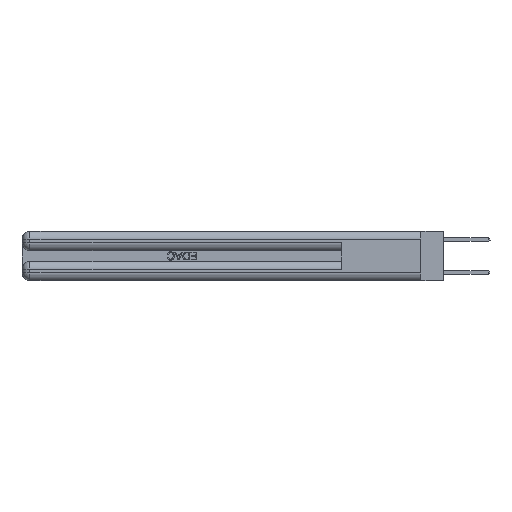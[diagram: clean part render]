
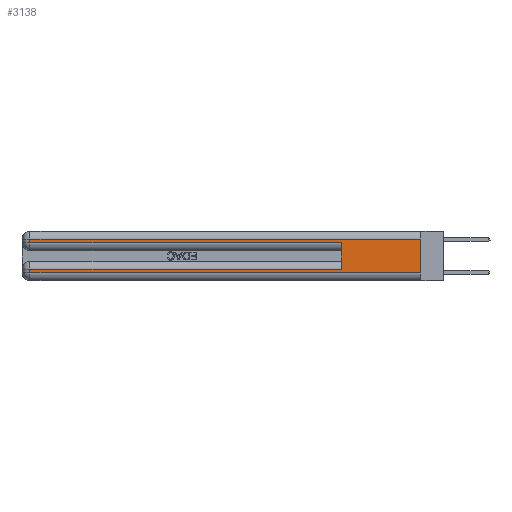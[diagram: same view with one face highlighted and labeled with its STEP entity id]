
A CAD part, left-side view. The second image highlights one B-rep face of the part: STEP entity #3138.
In plain terms, the highlighted planar face has unit normal (-1, 0, 0).
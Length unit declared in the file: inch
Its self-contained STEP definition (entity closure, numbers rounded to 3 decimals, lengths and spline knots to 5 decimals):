
#809 = VECTOR ( 'NONE', #23905, 39.37008 ) ;
#1511 = DIRECTION ( 'NONE',  ( 0., 1., 0. ) ) ;
#3138 = ADVANCED_FACE ( 'NONE', ( #25318 ), #23075, .F. ) ;
#3293 = LINE ( 'NONE', #7125, #24920 ) ;
#3451 = EDGE_CURVE ( 'NONE', #7905, #27086, #21387, .T. ) ;
#3602 = ORIENTED_EDGE ( 'NONE', *, *, #33795, .F. ) ;
#3707 = DIRECTION ( 'NONE',  ( 0., 0., -1. ) ) ;
#3880 = LINE ( 'NONE', #6873, #10560 ) ;
#3976 = CARTESIAN_POINT ( 'NONE',  ( 0., 2.94, 0.085 ) ) ;
#4169 = CARTESIAN_POINT ( 'NONE',  ( 0., 0., 0.285 ) ) ;
#4505 = VERTEX_POINT ( 'NONE', #17745 ) ;
#5614 = EDGE_CURVE ( 'NONE', #29169, #7905, #15104, .T. ) ;
#6213 = DIRECTION ( 'NONE',  ( 1., 0., 0. ) ) ;
#6358 = CARTESIAN_POINT ( 'NONE',  ( 0., 0., 0.06 ) ) ;
#6873 = CARTESIAN_POINT ( 'NONE',  ( 0., 2.94, 0.37 ) ) ;
#7125 = CARTESIAN_POINT ( 'NONE',  ( 0., 0., 0.31 ) ) ;
#7577 = VECTOR ( 'NONE', #28096, 39.37008 ) ;
#7658 = ORIENTED_EDGE ( 'NONE', *, *, #3451, .T. ) ;
#7905 = VERTEX_POINT ( 'NONE', #3976 ) ;
#7918 = EDGE_CURVE ( 'NONE', #4505, #29304, #3880, .T. ) ;
#8429 = ORIENTED_EDGE ( 'NONE', *, *, #30486, .T. ) ;
#9178 = DIRECTION ( 'NONE',  ( 0., -1., 0. ) ) ;
#9411 = CARTESIAN_POINT ( 'NONE',  ( 0., 0., 0.37 ) ) ;
#10560 = VECTOR ( 'NONE', #15416, 39.37008 ) ;
#11142 = CARTESIAN_POINT ( 'NONE',  ( 0., 0., 0.06 ) ) ;
#12797 = VERTEX_POINT ( 'NONE', #29211 ) ;
#13492 = LINE ( 'NONE', #6358, #29201 ) ;
#14343 = LINE ( 'NONE', #18410, #21787 ) ;
#14619 = LINE ( 'NONE', #9411, #22076 ) ;
#15104 = LINE ( 'NONE', #19707, #7577 ) ;
#15123 = CARTESIAN_POINT ( 'NONE',  ( 0., 0.6, 0.285 ) ) ;
#15416 = DIRECTION ( 'NONE',  ( 0., 0., -1. ) ) ;
#15652 = EDGE_CURVE ( 'NONE', #27086, #23393, #13492, .T. ) ;
#15997 = CARTESIAN_POINT ( 'NONE',  ( 0., 2.94, 0.37 ) ) ;
#17056 = ORIENTED_EDGE ( 'NONE', *, *, #18973, .F. ) ;
#17745 = CARTESIAN_POINT ( 'NONE',  ( 0., 2.94, 0.31 ) ) ;
#17817 = ORIENTED_EDGE ( 'NONE', *, *, #15652, .T. ) ;
#18156 = CARTESIAN_POINT ( 'NONE',  ( 0., 2.94, 0.06 ) ) ;
#18242 = AXIS2_PLACEMENT_3D ( 'NONE', #25750, #6213, #25868 ) ;
#18410 = CARTESIAN_POINT ( 'NONE',  ( 0., 0.6, 0.145 ) ) ;
#18891 = CARTESIAN_POINT ( 'NONE',  ( 0., 0.6, 0.085 ) ) ;
#18973 = EDGE_CURVE ( 'NONE', #12797, #23393, #14619, .T. ) ;
#19707 = CARTESIAN_POINT ( 'NONE',  ( 0., 0., 0.085 ) ) ;
#19783 = ORIENTED_EDGE ( 'NONE', *, *, #5614, .T. ) ;
#21387 = LINE ( 'NONE', #15997, #36224 ) ;
#21787 = VECTOR ( 'NONE', #22541, 39.37008 ) ;
#22076 = VECTOR ( 'NONE', #3707, 39.37008 ) ;
#22149 = ORIENTED_EDGE ( 'NONE', *, *, #7918, .T. ) ;
#22285 = CARTESIAN_POINT ( 'NONE',  ( 0., 2.94, 0.285 ) ) ;
#22541 = DIRECTION ( 'NONE',  ( 0., 0., 1. ) ) ;
#23075 = PLANE ( 'NONE',  #18242 ) ;
#23393 = VERTEX_POINT ( 'NONE', #11142 ) ;
#23905 = DIRECTION ( 'NONE',  ( 0., -1., 0. ) ) ;
#24920 = VECTOR ( 'NONE', #1511, 39.37008 ) ;
#25318 = FACE_OUTER_BOUND ( 'NONE', #30827, .T. ) ;
#25750 = CARTESIAN_POINT ( 'NONE',  ( 0., 0., 0.37 ) ) ;
#25868 = DIRECTION ( 'NONE',  ( 0., 0., -1. ) ) ;
#27086 = VERTEX_POINT ( 'NONE', #18156 ) ;
#27853 = EDGE_CURVE ( 'NONE', #12797, #4505, #3293, .T. ) ;
#28070 = ORIENTED_EDGE ( 'NONE', *, *, #27853, .T. ) ;
#28096 = DIRECTION ( 'NONE',  ( 0., 1., 0. ) ) ;
#28978 = LINE ( 'NONE', #4169, #809 ) ;
#29169 = VERTEX_POINT ( 'NONE', #18891 ) ;
#29201 = VECTOR ( 'NONE', #9178, 39.37008 ) ;
#29211 = CARTESIAN_POINT ( 'NONE',  ( 0., 0., 0.31 ) ) ;
#29304 = VERTEX_POINT ( 'NONE', #22285 ) ;
#30486 = EDGE_CURVE ( 'NONE', #29304, #36383, #28978, .T. ) ;
#30827 = EDGE_LOOP ( 'NONE', ( #17056, #28070, #22149, #8429, #3602, #19783, #7658, #17817 ) ) ;
#33795 = EDGE_CURVE ( 'NONE', #29169, #36383, #14343, .T. ) ;
#35525 = DIRECTION ( 'NONE',  ( 0., 0., -1. ) ) ;
#36224 = VECTOR ( 'NONE', #35525, 39.37008 ) ;
#36383 = VERTEX_POINT ( 'NONE', #15123 ) ;
